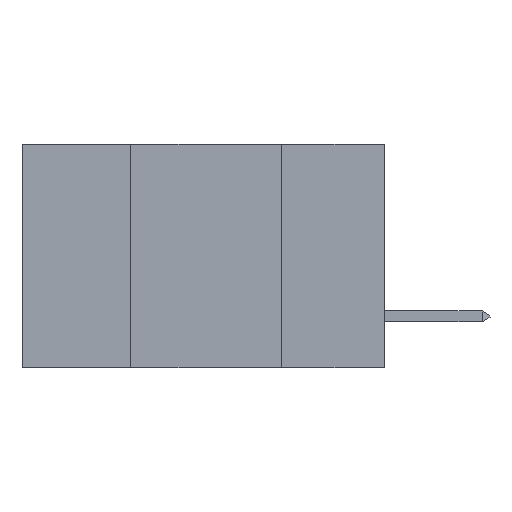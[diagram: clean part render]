
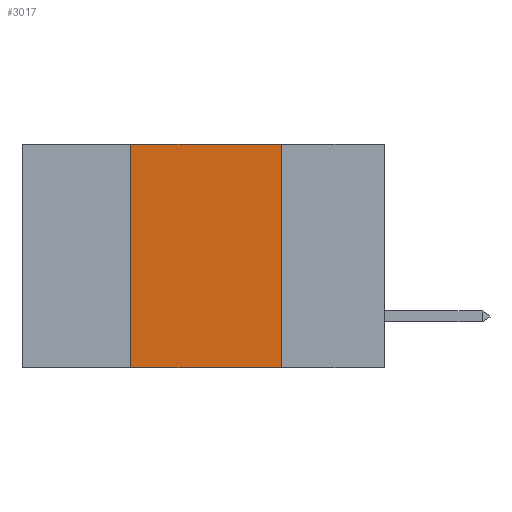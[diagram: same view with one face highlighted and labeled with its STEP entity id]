
A CAD part, left-side view. The second image highlights one B-rep face of the part: STEP entity #3017.
In plain terms, the highlighted planar face has unit normal (-1, 0, 0).
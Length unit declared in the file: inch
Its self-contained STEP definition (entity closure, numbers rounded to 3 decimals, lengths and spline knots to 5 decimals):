
#48 = ORIENTED_EDGE ( 'NONE', *, *, #1205, .F. ) ;
#163 = CARTESIAN_POINT ( 'NONE',  ( 0., 0.17, -0.37 ) ) ;
#752 = ORIENTED_EDGE ( 'NONE', *, *, #8554, .F. ) ;
#917 = CARTESIAN_POINT ( 'NONE',  ( 0., 0.17, 0. ) ) ;
#942 = VECTOR ( 'NONE', #7059, 39.37008 ) ;
#1180 = CARTESIAN_POINT ( 'NONE',  ( 0., 0.6, 0. ) ) ;
#1203 = VECTOR ( 'NONE', #3163, 39.37008 ) ;
#1205 = EDGE_CURVE ( 'NONE', #6962, #3190, #3364, .T. ) ;
#1367 = CARTESIAN_POINT ( 'NONE',  ( 0., 0.6, -0.37 ) ) ;
#2016 = CARTESIAN_POINT ( 'NONE',  ( 0., 0.42, -0.37 ) ) ;
#2872 = CARTESIAN_POINT ( 'NONE',  ( 0., 0.42, 0. ) ) ;
#3017 = ADVANCED_FACE ( 'NONE', ( #8643 ), #4042, .F. ) ;
#3163 = DIRECTION ( 'NONE',  ( 0., -1., 0. ) ) ;
#3190 = VERTEX_POINT ( 'NONE', #2872 ) ;
#3364 = LINE ( 'NONE', #7356, #6836 ) ;
#3482 = LINE ( 'NONE', #1367, #942 ) ;
#3897 = DIRECTION ( 'NONE',  ( 0., 0., -1. ) ) ;
#4042 = PLANE ( 'NONE',  #8173 ) ;
#4043 = EDGE_LOOP ( 'NONE', ( #752, #4346, #48, #4572 ) ) ;
#4323 = CARTESIAN_POINT ( 'NONE',  ( 0., 0.6, 0. ) ) ;
#4346 = ORIENTED_EDGE ( 'NONE', *, *, #5994, .F. ) ;
#4572 = ORIENTED_EDGE ( 'NONE', *, *, #8925, .T. ) ;
#4648 = VERTEX_POINT ( 'NONE', #163 ) ;
#4776 = CARTESIAN_POINT ( 'NONE',  ( 0., 0.17, 0. ) ) ;
#4960 = VECTOR ( 'NONE', #6099, 39.37008 ) ;
#5245 = DIRECTION ( 'NONE',  ( 1., 0., 0. ) ) ;
#5545 = DIRECTION ( 'NONE',  ( 0., 0., 1. ) ) ;
#5801 = VERTEX_POINT ( 'NONE', #4776 ) ;
#5994 = EDGE_CURVE ( 'NONE', #3190, #5801, #8612, .T. ) ;
#6099 = DIRECTION ( 'NONE',  ( 0., 0., -1. ) ) ;
#6552 = LINE ( 'NONE', #917, #4960 ) ;
#6836 = VECTOR ( 'NONE', #5545, 39.37008 ) ;
#6962 = VERTEX_POINT ( 'NONE', #2016 ) ;
#7059 = DIRECTION ( 'NONE',  ( 0., -1., 0. ) ) ;
#7356 = CARTESIAN_POINT ( 'NONE',  ( 0., 0.42, 0. ) ) ;
#8173 = AXIS2_PLACEMENT_3D ( 'NONE', #4323, #5245, #3897 ) ;
#8554 = EDGE_CURVE ( 'NONE', #5801, #4648, #6552, .T. ) ;
#8612 = LINE ( 'NONE', #1180, #1203 ) ;
#8643 = FACE_OUTER_BOUND ( 'NONE', #4043, .T. ) ;
#8925 = EDGE_CURVE ( 'NONE', #6962, #4648, #3482, .T. ) ;
